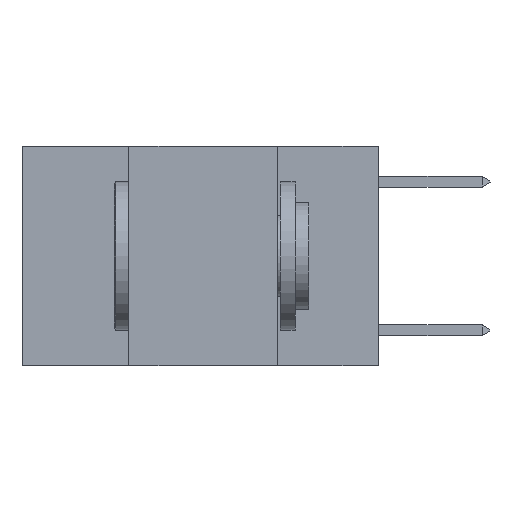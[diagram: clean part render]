
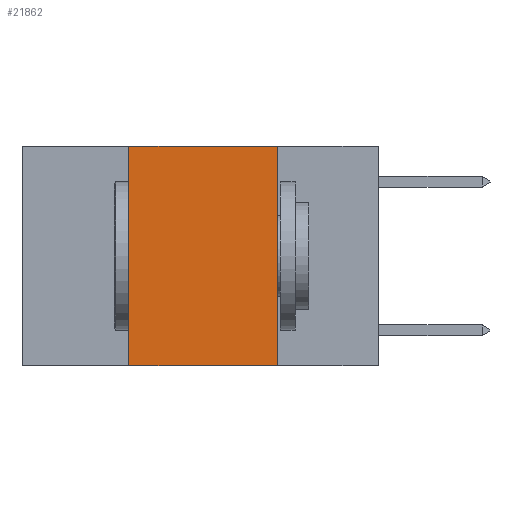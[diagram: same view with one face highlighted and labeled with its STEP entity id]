
A CAD part, left-side view. The second image highlights one B-rep face of the part: STEP entity #21862.
In plain terms, the highlighted planar face has unit normal (-1, 0, 0).
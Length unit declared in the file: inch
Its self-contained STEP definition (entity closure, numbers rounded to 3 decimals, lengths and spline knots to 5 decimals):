
#209 = VECTOR ( 'NONE', #17477, 39.37008 ) ;
#594 = DIRECTION ( 'NONE',  ( 0., 0., -1. ) ) ;
#711 = LINE ( 'NONE', #10235, #1760 ) ;
#910 = CARTESIAN_POINT ( 'NONE',  ( 0., 0.6, 0. ) ) ;
#1616 = EDGE_CURVE ( 'NONE', #3709, #7061, #711, .T. ) ;
#1619 = EDGE_CURVE ( 'NONE', #24440, #26969, #7904, .T. ) ;
#1668 = CARTESIAN_POINT ( 'NONE',  ( 0., 0.6, -0.37 ) ) ;
#1760 = VECTOR ( 'NONE', #19742, 39.37008 ) ;
#2207 = CARTESIAN_POINT ( 'NONE',  ( 0., 0.42, -0.37 ) ) ;
#3061 = VECTOR ( 'NONE', #6505, 39.37008 ) ;
#3709 = VERTEX_POINT ( 'NONE', #2207 ) ;
#5560 = CARTESIAN_POINT ( 'NONE',  ( 0., 0.17, 0. ) ) ;
#6505 = DIRECTION ( 'NONE',  ( 0., -1., 0. ) ) ;
#7061 = VERTEX_POINT ( 'NONE', #12623 ) ;
#7904 = LINE ( 'NONE', #5560, #9228 ) ;
#8104 = FACE_OUTER_BOUND ( 'NONE', #18667, .T. ) ;
#9228 = VECTOR ( 'NONE', #15684, 39.37008 ) ;
#10235 = CARTESIAN_POINT ( 'NONE',  ( 0., 0.42, 0. ) ) ;
#10447 = AXIS2_PLACEMENT_3D ( 'NONE', #910, #27138, #594 ) ;
#12623 = CARTESIAN_POINT ( 'NONE',  ( 0., 0.42, 0. ) ) ;
#12846 = EDGE_CURVE ( 'NONE', #7061, #24440, #26520, .T. ) ;
#15684 = DIRECTION ( 'NONE',  ( 0., 0., -1. ) ) ;
#16029 = ORIENTED_EDGE ( 'NONE', *, *, #1616, .F. ) ;
#16068 = CARTESIAN_POINT ( 'NONE',  ( 0., 0.17, -0.37 ) ) ;
#17477 = DIRECTION ( 'NONE',  ( 0., -1., 0. ) ) ;
#17616 = PLANE ( 'NONE',  #10447 ) ;
#18667 = EDGE_LOOP ( 'NONE', ( #24179, #29357, #16029, #22126 ) ) ;
#19420 = CARTESIAN_POINT ( 'NONE',  ( 0., 0.17, 0. ) ) ;
#19742 = DIRECTION ( 'NONE',  ( 0., 0., 1. ) ) ;
#21862 = ADVANCED_FACE ( 'NONE', ( #8104 ), #17616, .F. ) ;
#22126 = ORIENTED_EDGE ( 'NONE', *, *, #28572, .T. ) ;
#23050 = LINE ( 'NONE', #1668, #3061 ) ;
#24179 = ORIENTED_EDGE ( 'NONE', *, *, #1619, .F. ) ;
#24440 = VERTEX_POINT ( 'NONE', #19420 ) ;
#26520 = LINE ( 'NONE', #27144, #209 ) ;
#26969 = VERTEX_POINT ( 'NONE', #16068 ) ;
#27138 = DIRECTION ( 'NONE',  ( 1., 0., 0. ) ) ;
#27144 = CARTESIAN_POINT ( 'NONE',  ( 0., 0.6, 0. ) ) ;
#28572 = EDGE_CURVE ( 'NONE', #3709, #26969, #23050, .T. ) ;
#29357 = ORIENTED_EDGE ( 'NONE', *, *, #12846, .F. ) ;
